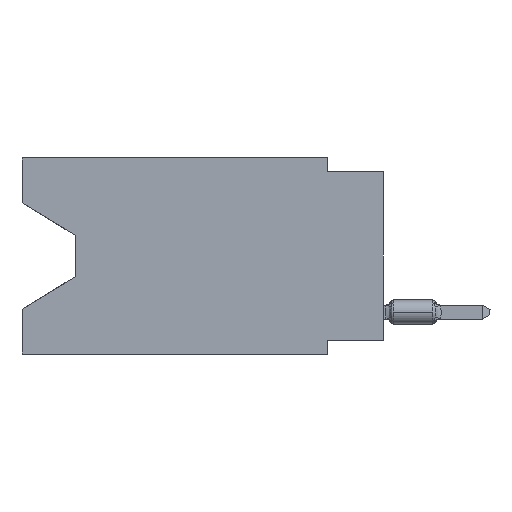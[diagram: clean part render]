
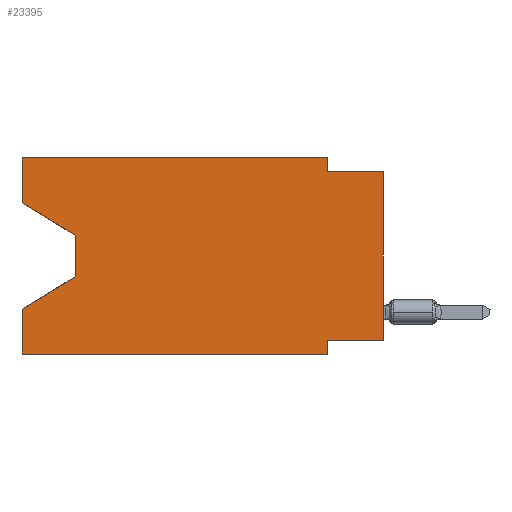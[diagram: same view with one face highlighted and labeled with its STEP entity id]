
A CAD part, left-side view. The second image highlights one B-rep face of the part: STEP entity #23395.
In plain terms, the highlighted planar face has unit normal (-1, 0, 0).
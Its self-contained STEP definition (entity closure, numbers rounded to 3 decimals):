
#274 = CARTESIAN_POINT ( 'NONE',  ( 0., 2.54, -8.89 ) ) ;
#377 = VERTEX_POINT ( 'NONE', #40372 ) ;
#463 = ORIENTED_EDGE ( 'NONE', *, *, #50813, .T. ) ;
#802 = DIRECTION ( 'NONE',  ( 0., -0.855, -0.519 ) ) ;
#1012 = CARTESIAN_POINT ( 'NONE',  ( 0., 16.383, 0. ) ) ;
#1792 = DIRECTION ( 'NONE',  ( 0., -1., 0. ) ) ;
#2072 = DIRECTION ( 'NONE',  ( 0., -1., 0. ) ) ;
#2229 = ORIENTED_EDGE ( 'NONE', *, *, #15971, .F. ) ;
#2653 = CARTESIAN_POINT ( 'NONE',  ( 0., 16.383, 0. ) ) ;
#5534 = DIRECTION ( 'NONE',  ( 0., 0., -1. ) ) ;
#5603 = LINE ( 'NONE', #51052, #27696 ) ;
#5648 = VECTOR ( 'NONE', #33141, 1000. ) ;
#6175 = EDGE_CURVE ( 'NONE', #20363, #19549, #30149, .T. ) ;
#6413 = EDGE_CURVE ( 'NONE', #30210, #377, #5603, .T. ) ;
#6419 = VECTOR ( 'NONE', #2072, 1000. ) ;
#6802 = CARTESIAN_POINT ( 'NONE',  ( 0., 13.97, -5.385 ) ) ;
#7031 = DIRECTION ( 'NONE',  ( 0., 1., 0. ) ) ;
#7215 = VECTOR ( 'NONE', #47567, 1000. ) ;
#7593 = AXIS2_PLACEMENT_3D ( 'NONE', #1012, #50280, #46737 ) ;
#7713 = EDGE_CURVE ( 'NONE', #45117, #8221, #36931, .T. ) ;
#8221 = VERTEX_POINT ( 'NONE', #25548 ) ;
#9594 = VERTEX_POINT ( 'NONE', #20853 ) ;
#10607 = ORIENTED_EDGE ( 'NONE', *, *, #7713, .F. ) ;
#11300 = ORIENTED_EDGE ( 'NONE', *, *, #6175, .T. ) ;
#12384 = LINE ( 'NONE', #6802, #58207 ) ;
#13652 = ORIENTED_EDGE ( 'NONE', *, *, #19273, .F. ) ;
#15424 = LINE ( 'NONE', #55550, #5648 ) ;
#15971 = EDGE_CURVE ( 'NONE', #20363, #39500, #52466, .T. ) ;
#16256 = EDGE_CURVE ( 'NONE', #9594, #23556, #54212, .T. ) ;
#17152 = CARTESIAN_POINT ( 'NONE',  ( 0., 0., 0. ) ) ;
#17326 = VECTOR ( 'NONE', #22473, 1000. ) ;
#17921 = EDGE_CURVE ( 'NONE', #45117, #22572, #54376, .T. ) ;
#19273 = EDGE_CURVE ( 'NONE', #9594, #35124, #29585, .T. ) ;
#19549 = VERTEX_POINT ( 'NONE', #50772 ) ;
#20363 = VERTEX_POINT ( 'NONE', #50552 ) ;
#20473 = CARTESIAN_POINT ( 'NONE',  ( 0., 13.97, -5.385 ) ) ;
#20677 = LINE ( 'NONE', #47241, #31550 ) ;
#20819 = ORIENTED_EDGE ( 'NONE', *, *, #6413, .F. ) ;
#20853 = CARTESIAN_POINT ( 'NONE',  ( 0., 16.383, -2.038 ) ) ;
#21012 = EDGE_CURVE ( 'NONE', #377, #19549, #51648, .T. ) ;
#22053 = ORIENTED_EDGE ( 'NONE', *, *, #24643, .F. ) ;
#22473 = DIRECTION ( 'NONE',  ( 0., 0., 1. ) ) ;
#22572 = VERTEX_POINT ( 'NONE', #274 ) ;
#23395 = ADVANCED_FACE ( 'NONE', ( #41434 ), #24023, .F. ) ;
#23556 = VERTEX_POINT ( 'NONE', #34898 ) ;
#24023 = PLANE ( 'NONE',  #7593 ) ;
#24643 = EDGE_CURVE ( 'NONE', #39500, #22572, #15424, .T. ) ;
#25548 = CARTESIAN_POINT ( 'NONE',  ( 0., 16.383, -6.852 ) ) ;
#25779 = ORIENTED_EDGE ( 'NONE', *, *, #32619, .T. ) ;
#25972 = CARTESIAN_POINT ( 'NONE',  ( 0., 2.54, -8.255 ) ) ;
#26020 = CARTESIAN_POINT ( 'NONE',  ( 0., 16.383, -8.89 ) ) ;
#27696 = VECTOR ( 'NONE', #41906, 1000. ) ;
#28007 = EDGE_LOOP ( 'NONE', ( #35630, #25779, #463, #10607, #37623, #22053, #2229, #11300, #40789, #20819, #47190, #13652 ) ) ;
#28118 = CARTESIAN_POINT ( 'NONE',  ( 0., 16.383, -8.89 ) ) ;
#28863 = CARTESIAN_POINT ( 'NONE',  ( 0., 13.97, -3.505 ) ) ;
#29585 = LINE ( 'NONE', #47003, #7215 ) ;
#30149 = LINE ( 'NONE', #17152, #17326 ) ;
#30210 = VERTEX_POINT ( 'NONE', #39484 ) ;
#30398 = DIRECTION ( 'NONE',  ( 0., 0.855, -0.519 ) ) ;
#31550 = VECTOR ( 'NONE', #1792, 1000. ) ;
#32503 = CARTESIAN_POINT ( 'NONE',  ( 0., 16.383, 0. ) ) ;
#32619 = EDGE_CURVE ( 'NONE', #23556, #53860, #37706, .T. ) ;
#33141 = DIRECTION ( 'NONE',  ( 0., 0., -1. ) ) ;
#33949 = CARTESIAN_POINT ( 'NONE',  ( 0., 0., -0.635 ) ) ;
#34898 = CARTESIAN_POINT ( 'NONE',  ( 0., 13.97, -3.505 ) ) ;
#35124 = VERTEX_POINT ( 'NONE', #2653 ) ;
#35630 = ORIENTED_EDGE ( 'NONE', *, *, #16256, .T. ) ;
#36508 = CARTESIAN_POINT ( 'NONE',  ( 0., 16.383, -2.038 ) ) ;
#36931 = LINE ( 'NONE', #32503, #56170 ) ;
#37623 = ORIENTED_EDGE ( 'NONE', *, *, #17921, .T. ) ;
#37706 = LINE ( 'NONE', #28863, #55773 ) ;
#39101 = VECTOR ( 'NONE', #7031, 1000. ) ;
#39484 = CARTESIAN_POINT ( 'NONE',  ( 0., 2.54, 0. ) ) ;
#39500 = VERTEX_POINT ( 'NONE', #25972 ) ;
#40372 = CARTESIAN_POINT ( 'NONE',  ( 0., 2.54, -0.635 ) ) ;
#40789 = ORIENTED_EDGE ( 'NONE', *, *, #21012, .F. ) ;
#41392 = DIRECTION ( 'NONE',  ( 0., -1., 0. ) ) ;
#41434 = FACE_OUTER_BOUND ( 'NONE', #28007, .T. ) ;
#41906 = DIRECTION ( 'NONE',  ( 0., 0., -1. ) ) ;
#42954 = VECTOR ( 'NONE', #802, 1000. ) ;
#43618 = CARTESIAN_POINT ( 'NONE',  ( 0., 0., -8.255 ) ) ;
#45117 = VERTEX_POINT ( 'NONE', #26020 ) ;
#45905 = VECTOR ( 'NONE', #41392, 1000. ) ;
#46084 = DIRECTION ( 'NONE',  ( 0., 0., 1. ) ) ;
#46737 = DIRECTION ( 'NONE',  ( 0., 0., -1. ) ) ;
#47003 = CARTESIAN_POINT ( 'NONE',  ( 0., 16.383, 0. ) ) ;
#47190 = ORIENTED_EDGE ( 'NONE', *, *, #47777, .F. ) ;
#47241 = CARTESIAN_POINT ( 'NONE',  ( 0., 16.383, 0. ) ) ;
#47567 = DIRECTION ( 'NONE',  ( 0., 0., 1. ) ) ;
#47777 = EDGE_CURVE ( 'NONE', #35124, #30210, #20677, .T. ) ;
#50280 = DIRECTION ( 'NONE',  ( 1., 0., 0. ) ) ;
#50552 = CARTESIAN_POINT ( 'NONE',  ( 0., 0., -8.255 ) ) ;
#50772 = CARTESIAN_POINT ( 'NONE',  ( 0., 0., -0.635 ) ) ;
#50813 = EDGE_CURVE ( 'NONE', #53860, #8221, #12384, .T. ) ;
#51052 = CARTESIAN_POINT ( 'NONE',  ( 0., 2.54, 0. ) ) ;
#51648 = LINE ( 'NONE', #33949, #6419 ) ;
#52466 = LINE ( 'NONE', #43618, #39101 ) ;
#53860 = VERTEX_POINT ( 'NONE', #20473 ) ;
#54212 = LINE ( 'NONE', #36508, #42954 ) ;
#54376 = LINE ( 'NONE', #28118, #45905 ) ;
#55550 = CARTESIAN_POINT ( 'NONE',  ( 0., 2.54, -8.89 ) ) ;
#55773 = VECTOR ( 'NONE', #5534, 1000. ) ;
#56170 = VECTOR ( 'NONE', #46084, 1000. ) ;
#58207 = VECTOR ( 'NONE', #30398, 1000. ) ;
